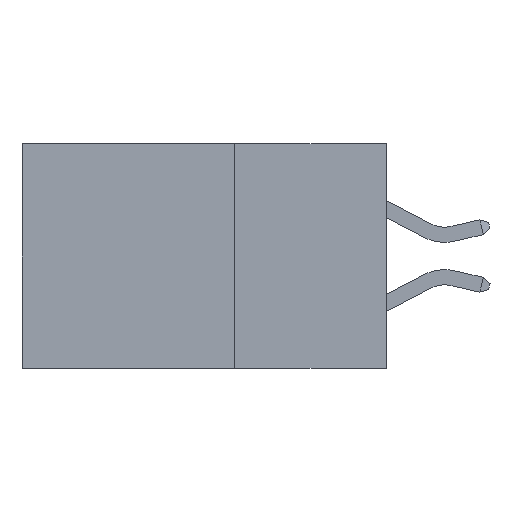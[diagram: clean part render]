
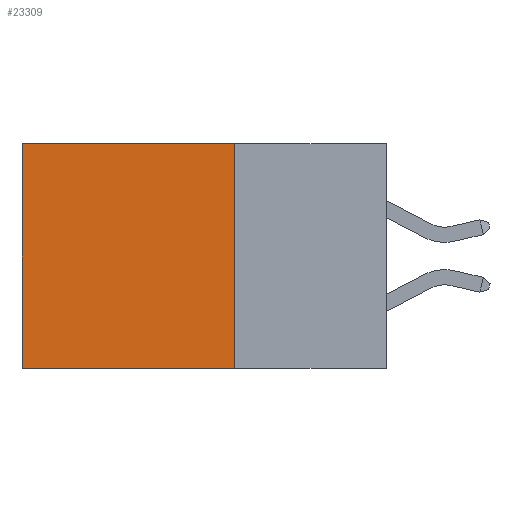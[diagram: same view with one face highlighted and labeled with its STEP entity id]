
A CAD part, left-side view. The second image highlights one B-rep face of the part: STEP entity #23309.
In plain terms, the highlighted planar face has unit normal (-1, 0, 0).
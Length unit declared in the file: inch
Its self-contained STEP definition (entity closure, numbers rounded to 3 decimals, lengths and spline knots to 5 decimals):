
#2 = PLANE ( 'NONE',  #13555 ) ;
#568 = VERTEX_POINT ( 'NONE', #5615 ) ;
#755 = DIRECTION ( 'NONE',  ( 0., 0., -1. ) ) ;
#1028 = CARTESIAN_POINT ( 'NONE',  ( 0.2615, 0.25, -0.37 ) ) ;
#2757 = DIRECTION ( 'NONE',  ( 0., 0., -1. ) ) ;
#3294 = EDGE_CURVE ( 'NONE', #4011, #10984, #18695, .T. ) ;
#3674 = DIRECTION ( 'NONE',  ( 0., 0., -1. ) ) ;
#3899 = EDGE_LOOP ( 'NONE', ( #17637, #6856, #20897, #12129 ) ) ;
#4011 = VERTEX_POINT ( 'NONE', #13430 ) ;
#5615 = CARTESIAN_POINT ( 'NONE',  ( 0.2615, 0.6, -0.37 ) ) ;
#6856 = ORIENTED_EDGE ( 'NONE', *, *, #13961, .F. ) ;
#6946 = CARTESIAN_POINT ( 'NONE',  ( 0.2615, 0.25, -0.37 ) ) ;
#7096 = CARTESIAN_POINT ( 'NONE',  ( 0.2615, 0.25, 0. ) ) ;
#7173 = DIRECTION ( 'NONE',  ( 0., 1., 0. ) ) ;
#7669 = VECTOR ( 'NONE', #8406, 39.37008 ) ;
#8298 = CARTESIAN_POINT ( 'NONE',  ( 0.2615, 0.25, -0.37 ) ) ;
#8406 = DIRECTION ( 'NONE',  ( 0., 1., 0. ) ) ;
#8723 = LINE ( 'NONE', #8298, #9863 ) ;
#9863 = VECTOR ( 'NONE', #2757, 39.37008 ) ;
#10984 = VERTEX_POINT ( 'NONE', #15233 ) ;
#11717 = CARTESIAN_POINT ( 'NONE',  ( 0.2615, 0.6, -0.37 ) ) ;
#12074 = VECTOR ( 'NONE', #755, 39.37008 ) ;
#12129 = ORIENTED_EDGE ( 'NONE', *, *, #3294, .T. ) ;
#12798 = CARTESIAN_POINT ( 'NONE',  ( 0.2615, 0.25, -0.37 ) ) ;
#13430 = CARTESIAN_POINT ( 'NONE',  ( 0.2615, 0.25, 0. ) ) ;
#13555 = AXIS2_PLACEMENT_3D ( 'NONE', #12798, #14654, #3674 ) ;
#13961 = EDGE_CURVE ( 'NONE', #22064, #568, #20808, .T. ) ;
#14654 = DIRECTION ( 'NONE',  ( 1., 0., 0. ) ) ;
#15130 = VECTOR ( 'NONE', #7173, 39.37008 ) ;
#15233 = CARTESIAN_POINT ( 'NONE',  ( 0.2615, 0.6, 0. ) ) ;
#15740 = LINE ( 'NONE', #11717, #12074 ) ;
#17637 = ORIENTED_EDGE ( 'NONE', *, *, #17715, .T. ) ;
#17715 = EDGE_CURVE ( 'NONE', #10984, #568, #15740, .T. ) ;
#18695 = LINE ( 'NONE', #7096, #15130 ) ;
#19767 = FACE_OUTER_BOUND ( 'NONE', #3899, .T. ) ;
#19830 = EDGE_CURVE ( 'NONE', #4011, #22064, #8723, .T. ) ;
#20808 = LINE ( 'NONE', #1028, #7669 ) ;
#20897 = ORIENTED_EDGE ( 'NONE', *, *, #19830, .F. ) ;
#22064 = VERTEX_POINT ( 'NONE', #6946 ) ;
#23309 = ADVANCED_FACE ( 'NONE', ( #19767 ), #2, .F. ) ;
